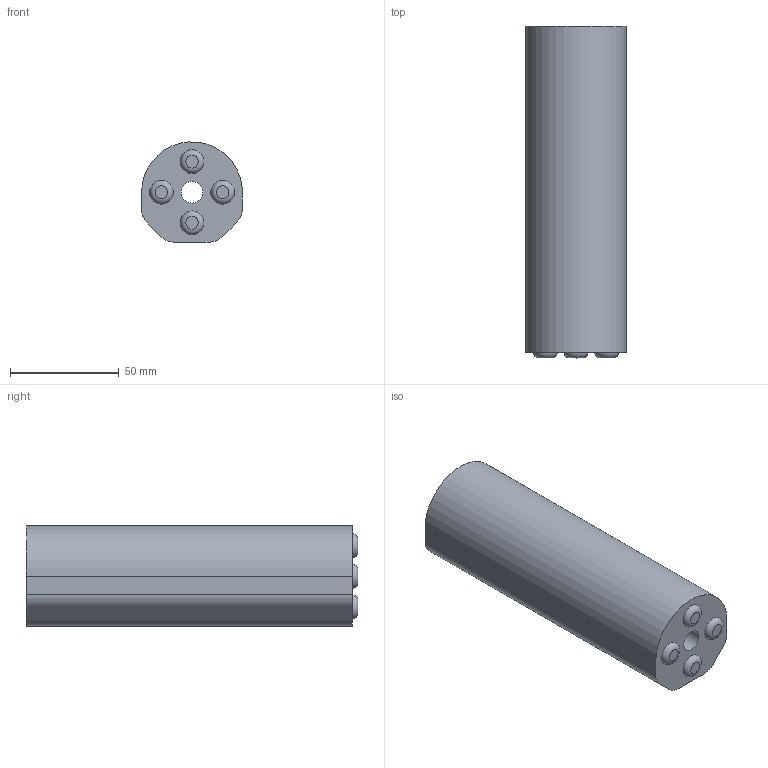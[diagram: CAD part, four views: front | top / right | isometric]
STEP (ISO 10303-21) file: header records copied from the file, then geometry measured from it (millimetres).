
FILE_DESCRIPTION((' '),'2;1');
FILE_NAME('Hydrabarrel2.stp','2013-06-04T21:39:49',(' '),(' '),' ','ACIS',' ');
FILE_SCHEMA(('CONFIG_CONTROL_DESIGN'));
Length unit declared in the file: inch
Products named in the file (1): Hydrabarrel2.stp
Bounding box: 46.28 x 152.4 x 45.93 mm (x, y, z)
Volume: 252238.1 mm3; surface area: 30858.2 mm2
Topology: 1 solids, 1 shells, 29 faces, 57 edges, 38 vertices
Faces by surface type: plane 15, cylinder 6, torus 4, bspline 4
Full cylindrical faces by diameter (mm): 9.906 x1
Entity records: 987 total; most frequent: CARTESIAN_POINT 292, DIRECTION 128, ORIENTED_EDGE 96, AXIS2_PLACEMENT_3D 54, EDGE_CURVE 48, EDGE_LOOP 48, VERTEX_POINT 38, FACE_OUTER_BOUND 29
